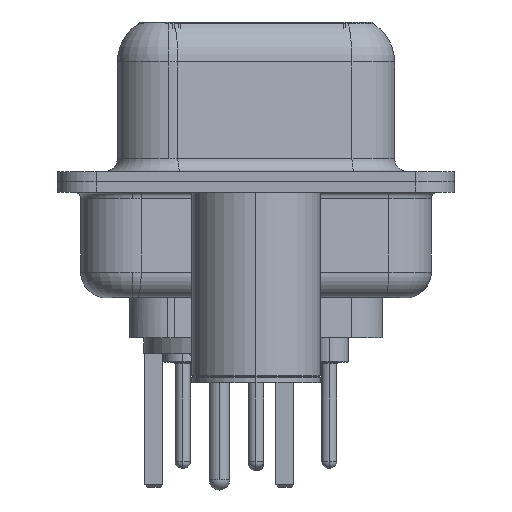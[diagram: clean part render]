
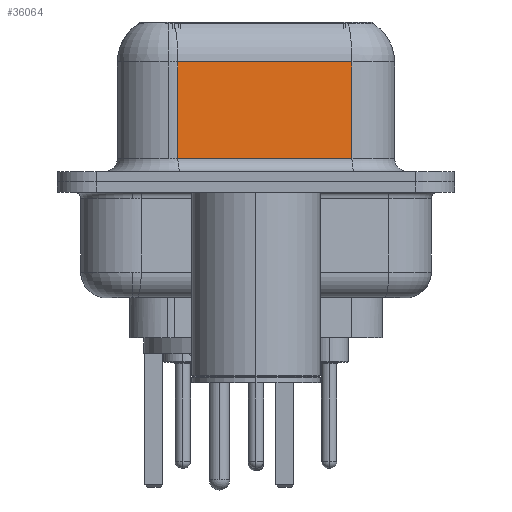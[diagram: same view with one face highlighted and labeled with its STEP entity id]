
A CAD part, left-side view. The second image highlights one B-rep face of the part: STEP entity #36064.
In plain terms, the highlighted planar face has unit normal (-0.985, -0.174, 0).
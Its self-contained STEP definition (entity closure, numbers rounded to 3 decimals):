
#1622 = VERTEX_POINT ( 'NONE', #17625 ) ;
#1857 = LINE ( 'NONE', #19984, #20089 ) ;
#1985 = VECTOR ( 'NONE', #25432, 1000. ) ;
#3408 = ORIENTED_EDGE ( 'NONE', *, *, #28914, .T. ) ;
#3606 = DIRECTION ( 'NONE',  ( 0.174, -0.985, 0. ) ) ;
#4508 = CARTESIAN_POINT ( 'NONE',  ( 4.43, 3.028, 4.65 ) ) ;
#4835 = AXIS2_PLACEMENT_3D ( 'NONE', #29359, #35040, #17900 ) ;
#5849 = VECTOR ( 'NONE', #28254, 1000. ) ;
#7916 = ORIENTED_EDGE ( 'NONE', *, *, #19468, .T. ) ;
#9119 = LINE ( 'NONE', #20346, #30837 ) ;
#10579 = VERTEX_POINT ( 'NONE', #4508 ) ;
#11817 = CARTESIAN_POINT ( 'NONE',  ( 5.621, -3.722, 4.65 ) ) ;
#13172 = VERTEX_POINT ( 'NONE', #14496 ) ;
#13359 = CARTESIAN_POINT ( 'NONE',  ( 4.43, 3.028, 0.9 ) ) ;
#14383 = DIRECTION ( 'NONE',  ( 0., 0., -1. ) ) ;
#14496 = CARTESIAN_POINT ( 'NONE',  ( 5.621, -3.722, 0.9 ) ) ;
#15065 = ORIENTED_EDGE ( 'NONE', *, *, #25066, .F. ) ;
#16707 = LINE ( 'NONE', #17266, #1985 ) ;
#16726 = VERTEX_POINT ( 'NONE', #13359 ) ;
#17266 = CARTESIAN_POINT ( 'NONE',  ( 5.621, -3.722, 6.4 ) ) ;
#17549 = EDGE_CURVE ( 'NONE', #1622, #10579, #35836, .T. ) ;
#17625 = CARTESIAN_POINT ( 'NONE',  ( 5.621, -3.722, 4.65 ) ) ;
#17900 = DIRECTION ( 'NONE',  ( -0.174, 0.985, 0. ) ) ;
#18268 = FACE_OUTER_BOUND ( 'NONE', #20920, .T. ) ;
#19468 = EDGE_CURVE ( 'NONE', #10579, #16726, #1857, .T. ) ;
#19984 = CARTESIAN_POINT ( 'NONE',  ( 4.43, 3.028, 6.4 ) ) ;
#20089 = VECTOR ( 'NONE', #14383, 1000. ) ;
#20346 = CARTESIAN_POINT ( 'NONE',  ( 5.621, -3.722, 0.9 ) ) ;
#20920 = EDGE_LOOP ( 'NONE', ( #15065, #32229, #7916, #3408 ) ) ;
#20937 = PLANE ( 'NONE',  #4835 ) ;
#25066 = EDGE_CURVE ( 'NONE', #1622, #13172, #16707, .T. ) ;
#25432 = DIRECTION ( 'NONE',  ( 0., 0., -1. ) ) ;
#28254 = DIRECTION ( 'NONE',  ( -0.174, 0.985, 0. ) ) ;
#28914 = EDGE_CURVE ( 'NONE', #16726, #13172, #9119, .T. ) ;
#29359 = CARTESIAN_POINT ( 'NONE',  ( 5.621, -3.722, 6.4 ) ) ;
#30837 = VECTOR ( 'NONE', #3606, 1000. ) ;
#32229 = ORIENTED_EDGE ( 'NONE', *, *, #17549, .T. ) ;
#35040 = DIRECTION ( 'NONE',  ( 0.985, 0.174, 0. ) ) ;
#35836 = LINE ( 'NONE', #11817, #5849 ) ;
#36064 = ADVANCED_FACE ( 'NONE', ( #18268 ), #20937, .F. ) ;
